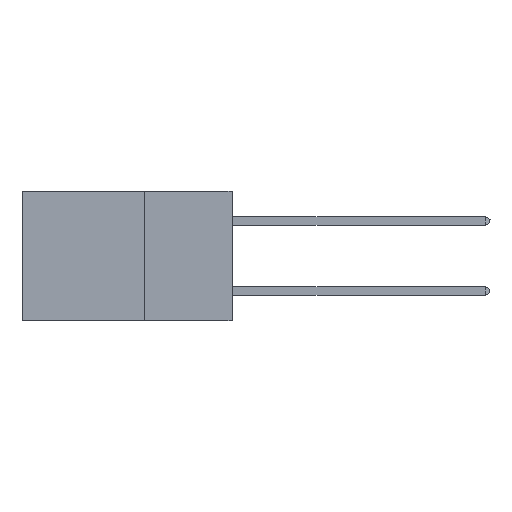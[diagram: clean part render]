
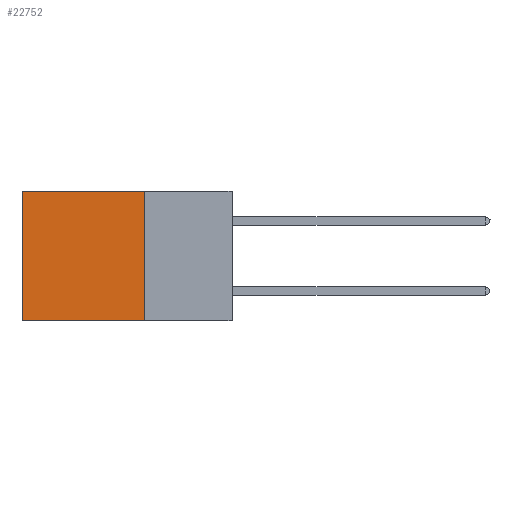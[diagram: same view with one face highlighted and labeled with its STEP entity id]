
A CAD part, left-side view. The second image highlights one B-rep face of the part: STEP entity #22752.
In plain terms, the highlighted planar face has unit normal (-1, 0, 0).
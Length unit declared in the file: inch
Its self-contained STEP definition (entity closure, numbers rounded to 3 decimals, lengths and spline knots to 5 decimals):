
#92 = VERTEX_POINT ( 'NONE', #18101 ) ;
#366 = CARTESIAN_POINT ( 'NONE',  ( 0.2875, 0.6, 0. ) ) ;
#826 = EDGE_CURVE ( 'NONE', #1792, #92, #21004, .T. ) ;
#1057 = CARTESIAN_POINT ( 'NONE',  ( 0.2875, 0.25, -0.37 ) ) ;
#1168 = LINE ( 'NONE', #3172, #7716 ) ;
#1435 = DIRECTION ( 'NONE',  ( 0., 1., 0. ) ) ;
#1792 = VERTEX_POINT ( 'NONE', #6293 ) ;
#2010 = LINE ( 'NONE', #13586, #5515 ) ;
#3172 = CARTESIAN_POINT ( 'NONE',  ( 0.2875, 0.25, 0. ) ) ;
#3357 = CARTESIAN_POINT ( 'NONE',  ( 0.2875, 0.25, 0. ) ) ;
#5412 = ORIENTED_EDGE ( 'NONE', *, *, #826, .F. ) ;
#5515 = VECTOR ( 'NONE', #9877, 39.37008 ) ;
#6293 = CARTESIAN_POINT ( 'NONE',  ( 0.2875, 0.25, -0.37 ) ) ;
#6380 = VECTOR ( 'NONE', #18981, 39.37008 ) ;
#6402 = PLANE ( 'NONE',  #11698 ) ;
#6591 = EDGE_CURVE ( 'NONE', #7534, #8085, #1168, .T. ) ;
#7264 = ORIENTED_EDGE ( 'NONE', *, *, #6591, .T. ) ;
#7534 = VERTEX_POINT ( 'NONE', #3357 ) ;
#7716 = VECTOR ( 'NONE', #1435, 39.37008 ) ;
#8085 = VERTEX_POINT ( 'NONE', #366 ) ;
#8665 = DIRECTION ( 'NONE',  ( 0., 0., -1. ) ) ;
#8789 = LINE ( 'NONE', #12626, #14579 ) ;
#9624 = EDGE_CURVE ( 'NONE', #8085, #92, #8789, .T. ) ;
#9877 = DIRECTION ( 'NONE',  ( 0., 0., -1. ) ) ;
#11698 = AXIS2_PLACEMENT_3D ( 'NONE', #16349, #22473, #14096 ) ;
#12297 = EDGE_CURVE ( 'NONE', #7534, #1792, #2010, .T. ) ;
#12626 = CARTESIAN_POINT ( 'NONE',  ( 0.2875, 0.6, 0. ) ) ;
#13586 = CARTESIAN_POINT ( 'NONE',  ( 0.2875, 0.25, 0. ) ) ;
#14096 = DIRECTION ( 'NONE',  ( 0., 0., -1. ) ) ;
#14233 = FACE_OUTER_BOUND ( 'NONE', #14708, .T. ) ;
#14579 = VECTOR ( 'NONE', #8665, 39.37008 ) ;
#14708 = EDGE_LOOP ( 'NONE', ( #22652, #5412, #20034, #7264 ) ) ;
#16349 = CARTESIAN_POINT ( 'NONE',  ( 0.2875, 0.25, 0. ) ) ;
#18101 = CARTESIAN_POINT ( 'NONE',  ( 0.2875, 0.6, -0.37 ) ) ;
#18981 = DIRECTION ( 'NONE',  ( 0., 1., 0. ) ) ;
#20034 = ORIENTED_EDGE ( 'NONE', *, *, #12297, .F. ) ;
#21004 = LINE ( 'NONE', #1057, #6380 ) ;
#22473 = DIRECTION ( 'NONE',  ( 1., 0., 0. ) ) ;
#22652 = ORIENTED_EDGE ( 'NONE', *, *, #9624, .T. ) ;
#22752 = ADVANCED_FACE ( 'NONE', ( #14233 ), #6402, .F. ) ;
